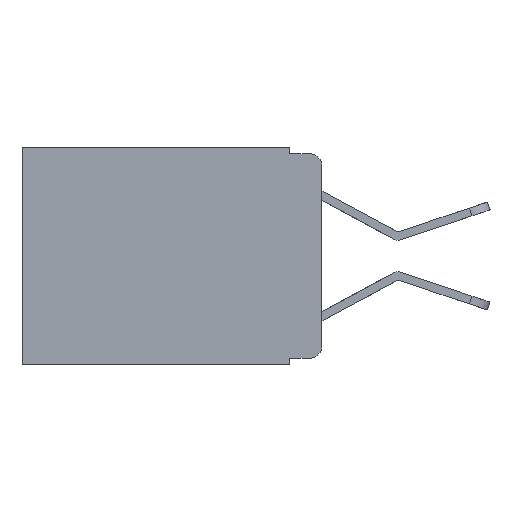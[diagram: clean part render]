
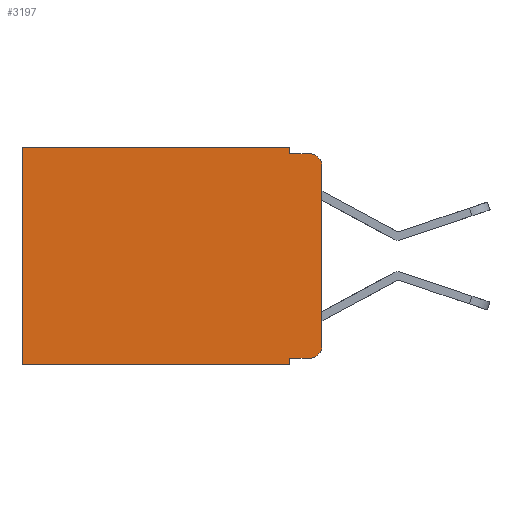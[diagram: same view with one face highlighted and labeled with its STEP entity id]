
A CAD part, left-side view. The second image highlights one B-rep face of the part: STEP entity #3197.
In plain terms, the highlighted planar face has unit normal (-1, 0, 0).
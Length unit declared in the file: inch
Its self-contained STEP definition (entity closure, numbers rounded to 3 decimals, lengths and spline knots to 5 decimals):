
#71 = CARTESIAN_POINT ( 'NONE',  ( 0.298, 0.02, -0.01 ) ) ;
#74 = ORIENTED_EDGE ( 'NONE', *, *, #5121, .F. ) ;
#80 = LINE ( 'NONE', #9665, #10966 ) ;
#692 = VECTOR ( 'NONE', #10186, 39.37008 ) ;
#965 = ORIENTED_EDGE ( 'NONE', *, *, #3629, .F. ) ;
#1012 = VERTEX_POINT ( 'NONE', #10971 ) ;
#1086 = CARTESIAN_POINT ( 'NONE',  ( 0.298, 0.051, -0.333 ) ) ;
#1294 = LINE ( 'NONE', #5292, #5686 ) ;
#1424 = VERTEX_POINT ( 'NONE', #71 ) ;
#1617 = ORIENTED_EDGE ( 'NONE', *, *, #6310, .T. ) ;
#1979 = EDGE_CURVE ( 'NONE', #6442, #1424, #8497, .T. ) ;
#2141 = ORIENTED_EDGE ( 'NONE', *, *, #8201, .T. ) ;
#2148 = CARTESIAN_POINT ( 'NONE',  ( 0.298, 0.02, -0.313 ) ) ;
#3024 = VECTOR ( 'NONE', #8032, 39.37008 ) ;
#3045 = DIRECTION ( 'NONE',  ( 0., 0., -1. ) ) ;
#3197 = ADVANCED_FACE ( 'NONE', ( #3544 ), #9374, .F. ) ;
#3260 = EDGE_CURVE ( 'NONE', #8443, #4409, #9762, .T. ) ;
#3523 = DIRECTION ( 'NONE',  ( 0., 0., -1. ) ) ;
#3544 = FACE_OUTER_BOUND ( 'NONE', #8002, .T. ) ;
#3629 = EDGE_CURVE ( 'NONE', #10695, #9212, #8081, .T. ) ;
#3726 = CARTESIAN_POINT ( 'NONE',  ( 0.298, 0.051, 0. ) ) ;
#3745 = CARTESIAN_POINT ( 'NONE',  ( 0.298, 0.02, -0.333 ) ) ;
#3855 = CARTESIAN_POINT ( 'NONE',  ( 0.298, 0.473, 0. ) ) ;
#3915 = ORIENTED_EDGE ( 'NONE', *, *, #1979, .F. ) ;
#4060 = CARTESIAN_POINT ( 'NONE',  ( 0.298, 0.051, -0.01 ) ) ;
#4409 = VERTEX_POINT ( 'NONE', #9315 ) ;
#4616 = DIRECTION ( 'NONE',  ( 0., 0., -1. ) ) ;
#4630 = CARTESIAN_POINT ( 'NONE',  ( 0.298, 0., 0. ) ) ;
#4677 = CARTESIAN_POINT ( 'NONE',  ( 0.298, 0.02, -0.03 ) ) ;
#4736 = CARTESIAN_POINT ( 'NONE',  ( 0.298, 0., 0. ) ) ;
#4869 = ORIENTED_EDGE ( 'NONE', *, *, #9590, .F. ) ;
#5043 = CIRCLE ( 'NONE', #7124, 0.02 ) ;
#5121 = EDGE_CURVE ( 'NONE', #5966, #5700, #9775, .T. ) ;
#5172 = CARTESIAN_POINT ( 'NONE',  ( 0.298, 0.051, -0.333 ) ) ;
#5211 = ORIENTED_EDGE ( 'NONE', *, *, #7279, .F. ) ;
#5292 = CARTESIAN_POINT ( 'NONE',  ( 0.298, 0., -0.343 ) ) ;
#5471 = CARTESIAN_POINT ( 'NONE',  ( 0.298, 0.051, -0.01 ) ) ;
#5511 = DIRECTION ( 'NONE',  ( 0., 1., 0. ) ) ;
#5557 = DIRECTION ( 'NONE',  ( 0., 0., -1. ) ) ;
#5686 = VECTOR ( 'NONE', #6149, 39.37008 ) ;
#5700 = VERTEX_POINT ( 'NONE', #8758 ) ;
#5966 = VERTEX_POINT ( 'NONE', #9952 ) ;
#6149 = DIRECTION ( 'NONE',  ( 0., 1., 0. ) ) ;
#6218 = EDGE_CURVE ( 'NONE', #1012, #8443, #6649, .T. ) ;
#6277 = VECTOR ( 'NONE', #9034, 39.37008 ) ;
#6310 = EDGE_CURVE ( 'NONE', #7404, #5700, #5043, .T. ) ;
#6327 = DIRECTION ( 'NONE',  ( 0., 0., -1. ) ) ;
#6396 = DIRECTION ( 'NONE',  ( 1., 0., 0. ) ) ;
#6442 = VERTEX_POINT ( 'NONE', #4060 ) ;
#6474 = AXIS2_PLACEMENT_3D ( 'NONE', #4736, #6396, #6327 ) ;
#6649 = LINE ( 'NONE', #4630, #7822 ) ;
#7059 = ORIENTED_EDGE ( 'NONE', *, *, #10724, .T. ) ;
#7124 = AXIS2_PLACEMENT_3D ( 'NONE', #2148, #8161, #3045 ) ;
#7279 = EDGE_CURVE ( 'NONE', #9212, #4409, #1294, .T. ) ;
#7404 = VERTEX_POINT ( 'NONE', #3745 ) ;
#7446 = ORIENTED_EDGE ( 'NONE', *, *, #6218, .T. ) ;
#7627 = LINE ( 'NONE', #5172, #692 ) ;
#7822 = VECTOR ( 'NONE', #5511, 39.37008 ) ;
#8002 = EDGE_LOOP ( 'NONE', ( #74, #7059, #3915, #4869, #7446, #8718, #5211, #965, #2141, #1617 ) ) ;
#8032 = DIRECTION ( 'NONE',  ( 0., 0., -1. ) ) ;
#8081 = LINE ( 'NONE', #3726, #10268 ) ;
#8161 = DIRECTION ( 'NONE',  ( -1., 0., 0. ) ) ;
#8201 = EDGE_CURVE ( 'NONE', #10695, #7404, #7627, .T. ) ;
#8266 = CARTESIAN_POINT ( 'NONE',  ( 0.298, 0.051, -0.343 ) ) ;
#8443 = VERTEX_POINT ( 'NONE', #3855 ) ;
#8497 = LINE ( 'NONE', #5471, #6277 ) ;
#8718 = ORIENTED_EDGE ( 'NONE', *, *, #3260, .T. ) ;
#8758 = CARTESIAN_POINT ( 'NONE',  ( 0.298, 0., -0.313 ) ) ;
#8888 = CARTESIAN_POINT ( 'NONE',  ( 0.298, 0., 0. ) ) ;
#9034 = DIRECTION ( 'NONE',  ( 0., -1., 0. ) ) ;
#9115 = AXIS2_PLACEMENT_3D ( 'NONE', #4677, #10546, #5557 ) ;
#9130 = CARTESIAN_POINT ( 'NONE',  ( 0.298, 0.473, 0. ) ) ;
#9173 = DIRECTION ( 'NONE',  ( 0., 0., -1. ) ) ;
#9212 = VERTEX_POINT ( 'NONE', #8266 ) ;
#9315 = CARTESIAN_POINT ( 'NONE',  ( 0.298, 0.473, -0.343 ) ) ;
#9374 = PLANE ( 'NONE',  #6474 ) ;
#9517 = VECTOR ( 'NONE', #9173, 39.37008 ) ;
#9590 = EDGE_CURVE ( 'NONE', #1012, #6442, #80, .T. ) ;
#9665 = CARTESIAN_POINT ( 'NONE',  ( 0.298, 0.051, 0. ) ) ;
#9762 = LINE ( 'NONE', #9130, #9517 ) ;
#9775 = LINE ( 'NONE', #8888, #3024 ) ;
#9952 = CARTESIAN_POINT ( 'NONE',  ( 0.298, 0., -0.03 ) ) ;
#9982 = CIRCLE ( 'NONE', #9115, 0.02 ) ;
#10186 = DIRECTION ( 'NONE',  ( 0., -1., 0. ) ) ;
#10268 = VECTOR ( 'NONE', #3523, 39.37008 ) ;
#10546 = DIRECTION ( 'NONE',  ( -1., 0., 0. ) ) ;
#10695 = VERTEX_POINT ( 'NONE', #1086 ) ;
#10724 = EDGE_CURVE ( 'NONE', #5966, #1424, #9982, .T. ) ;
#10966 = VECTOR ( 'NONE', #4616, 39.37008 ) ;
#10971 = CARTESIAN_POINT ( 'NONE',  ( 0.298, 0.051, 0. ) ) ;
